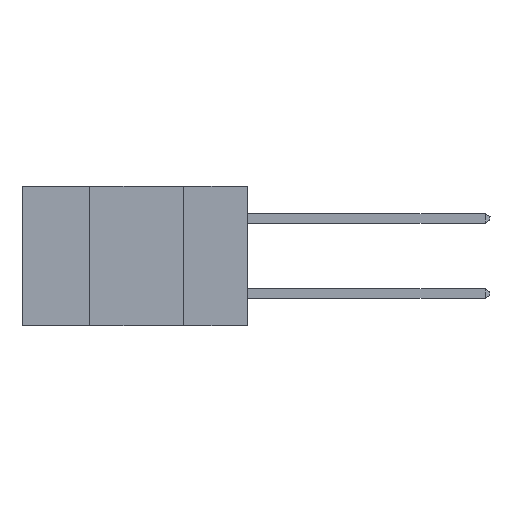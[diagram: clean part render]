
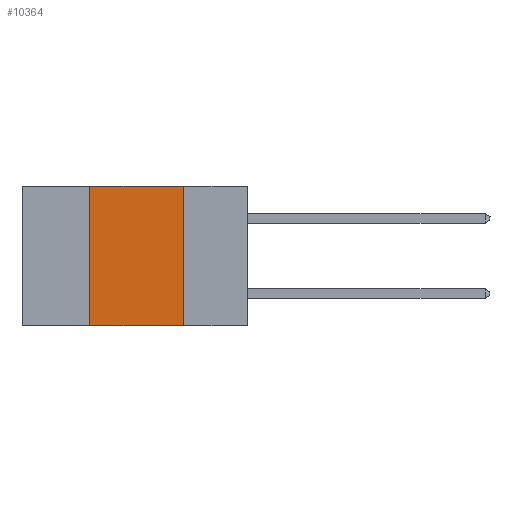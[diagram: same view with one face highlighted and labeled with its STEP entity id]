
A CAD part, left-side view. The second image highlights one B-rep face of the part: STEP entity #10364.
In plain terms, the highlighted planar face has unit normal (-1, 0, 0).
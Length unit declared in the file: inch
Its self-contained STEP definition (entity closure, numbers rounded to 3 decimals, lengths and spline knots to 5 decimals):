
#770 = LINE ( 'NONE', #21325, #12014 ) ;
#1066 = VECTOR ( 'NONE', #8883, 39.37008 ) ;
#1228 = VERTEX_POINT ( 'NONE', #21469 ) ;
#2778 = EDGE_CURVE ( 'NONE', #10255, #1228, #3402, .T. ) ;
#3402 = LINE ( 'NONE', #23449, #8866 ) ;
#3898 = FACE_OUTER_BOUND ( 'NONE', #13494, .T. ) ;
#5821 = VERTEX_POINT ( 'NONE', #23852 ) ;
#6433 = AXIS2_PLACEMENT_3D ( 'NONE', #18916, #13230, #22353 ) ;
#7662 = CARTESIAN_POINT ( 'NONE',  ( 0., 0.42, -0.37 ) ) ;
#8866 = VECTOR ( 'NONE', #21983, 39.37008 ) ;
#8883 = DIRECTION ( 'NONE',  ( 0., 0., 1. ) ) ;
#10185 = ORIENTED_EDGE ( 'NONE', *, *, #15030, .T. ) ;
#10255 = VERTEX_POINT ( 'NONE', #19578 ) ;
#10364 = ADVANCED_FACE ( 'NONE', ( #3898 ), #11386, .F. ) ;
#11027 = ORIENTED_EDGE ( 'NONE', *, *, #21649, .F. ) ;
#11386 = PLANE ( 'NONE',  #6433 ) ;
#12014 = VECTOR ( 'NONE', #19233, 39.37008 ) ;
#13230 = DIRECTION ( 'NONE',  ( 1., 0., 0. ) ) ;
#13494 = EDGE_LOOP ( 'NONE', ( #11027, #21378, #18995, #10185 ) ) ;
#14025 = VECTOR ( 'NONE', #23955, 39.37008 ) ;
#14930 = VERTEX_POINT ( 'NONE', #7662 ) ;
#15030 = EDGE_CURVE ( 'NONE', #14930, #5821, #770, .T. ) ;
#16046 = LINE ( 'NONE', #16175, #1066 ) ;
#16175 = CARTESIAN_POINT ( 'NONE',  ( 0., 0.42, -0.37 ) ) ;
#18438 = CARTESIAN_POINT ( 'NONE',  ( 0., 0.17, -0.37 ) ) ;
#18916 = CARTESIAN_POINT ( 'NONE',  ( 0., 0.6, 0. ) ) ;
#18995 = ORIENTED_EDGE ( 'NONE', *, *, #19295, .F. ) ;
#19233 = DIRECTION ( 'NONE',  ( 0., -1., 0. ) ) ;
#19295 = EDGE_CURVE ( 'NONE', #14930, #10255, #16046, .T. ) ;
#19578 = CARTESIAN_POINT ( 'NONE',  ( 0., 0.42, 0. ) ) ;
#20649 = LINE ( 'NONE', #18438, #14025 ) ;
#21325 = CARTESIAN_POINT ( 'NONE',  ( 0., 0.6, -0.37 ) ) ;
#21378 = ORIENTED_EDGE ( 'NONE', *, *, #2778, .F. ) ;
#21469 = CARTESIAN_POINT ( 'NONE',  ( 0., 0.17, 0. ) ) ;
#21649 = EDGE_CURVE ( 'NONE', #1228, #5821, #20649, .T. ) ;
#21983 = DIRECTION ( 'NONE',  ( 0., -1., 0. ) ) ;
#22353 = DIRECTION ( 'NONE',  ( 0., 0., -1. ) ) ;
#23449 = CARTESIAN_POINT ( 'NONE',  ( 0., 0.6, 0. ) ) ;
#23852 = CARTESIAN_POINT ( 'NONE',  ( 0., 0.17, -0.37 ) ) ;
#23955 = DIRECTION ( 'NONE',  ( 0., 0., -1. ) ) ;
